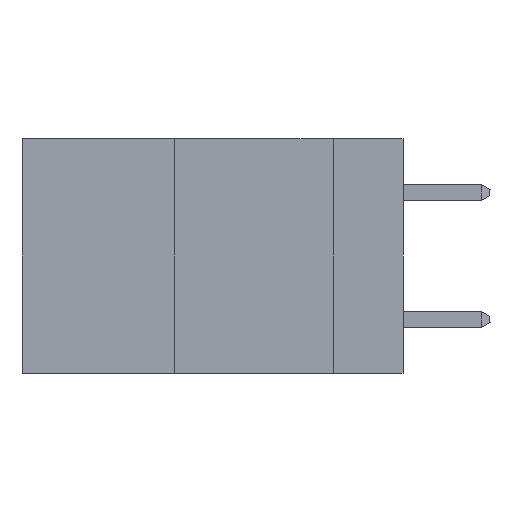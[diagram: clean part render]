
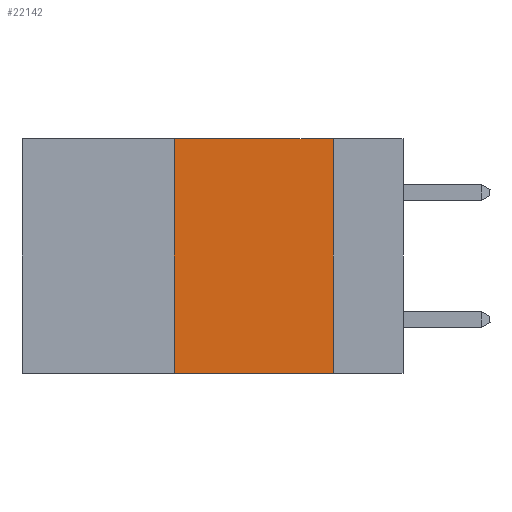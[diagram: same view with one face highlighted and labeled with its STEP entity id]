
A CAD part, left-side view. The second image highlights one B-rep face of the part: STEP entity #22142.
In plain terms, the highlighted planar face has unit normal (-1, 0, 0).
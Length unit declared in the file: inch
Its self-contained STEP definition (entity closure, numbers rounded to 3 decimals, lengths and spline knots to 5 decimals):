
#327 = EDGE_LOOP ( 'NONE', ( #36413, #17325, #36141, #30647 ) ) ;
#2615 = AXIS2_PLACEMENT_3D ( 'NONE', #5305, #29516, #26324 ) ;
#3055 = EDGE_CURVE ( 'NONE', #9869, #35021, #11047, .T. ) ;
#5305 = CARTESIAN_POINT ( 'NONE',  ( 0., 0.6, 0. ) ) ;
#6634 = EDGE_CURVE ( 'NONE', #38166, #34786, #30590, .T. ) ;
#7821 = CARTESIAN_POINT ( 'NONE',  ( 0., 0.11, -0.37 ) ) ;
#8648 = CARTESIAN_POINT ( 'NONE',  ( 0., 0.36, 0. ) ) ;
#9847 = DIRECTION ( 'NONE',  ( 0., 0., 1. ) ) ;
#9869 = VERTEX_POINT ( 'NONE', #22247 ) ;
#10878 = DIRECTION ( 'NONE',  ( 0., 0., -1. ) ) ;
#11047 = LINE ( 'NONE', #19225, #32716 ) ;
#12636 = DIRECTION ( 'NONE',  ( 0., -1., 0. ) ) ;
#12850 = FACE_OUTER_BOUND ( 'NONE', #327, .T. ) ;
#17325 = ORIENTED_EDGE ( 'NONE', *, *, #6634, .F. ) ;
#18209 = EDGE_CURVE ( 'NONE', #34786, #35021, #38757, .T. ) ;
#18519 = DIRECTION ( 'NONE',  ( 0., -1., 0. ) ) ;
#19225 = CARTESIAN_POINT ( 'NONE',  ( 0., 0.6, -0.37 ) ) ;
#19357 = CARTESIAN_POINT ( 'NONE',  ( 0., 0.6, 0. ) ) ;
#20400 = PLANE ( 'NONE',  #2615 ) ;
#22039 = VECTOR ( 'NONE', #18519, 39.37008 ) ;
#22142 = ADVANCED_FACE ( 'NONE', ( #12850 ), #20400, .F. ) ;
#22247 = CARTESIAN_POINT ( 'NONE',  ( 0., 0.36, -0.37 ) ) ;
#22676 = VECTOR ( 'NONE', #10878, 39.37008 ) ;
#23154 = CARTESIAN_POINT ( 'NONE',  ( 0., 0.11, 0. ) ) ;
#26324 = DIRECTION ( 'NONE',  ( 0., 0., -1. ) ) ;
#28230 = CARTESIAN_POINT ( 'NONE',  ( 0., 0.36, 0. ) ) ;
#29516 = DIRECTION ( 'NONE',  ( 1., 0., 0. ) ) ;
#30590 = LINE ( 'NONE', #19357, #22039 ) ;
#30647 = ORIENTED_EDGE ( 'NONE', *, *, #3055, .T. ) ;
#31687 = LINE ( 'NONE', #28230, #37787 ) ;
#32716 = VECTOR ( 'NONE', #12636, 39.37008 ) ;
#33548 = CARTESIAN_POINT ( 'NONE',  ( 0., 0.11, 0. ) ) ;
#33868 = EDGE_CURVE ( 'NONE', #9869, #38166, #31687, .T. ) ;
#34786 = VERTEX_POINT ( 'NONE', #33548 ) ;
#35021 = VERTEX_POINT ( 'NONE', #7821 ) ;
#36141 = ORIENTED_EDGE ( 'NONE', *, *, #33868, .F. ) ;
#36413 = ORIENTED_EDGE ( 'NONE', *, *, #18209, .F. ) ;
#37787 = VECTOR ( 'NONE', #9847, 39.37008 ) ;
#38166 = VERTEX_POINT ( 'NONE', #8648 ) ;
#38757 = LINE ( 'NONE', #23154, #22676 ) ;
